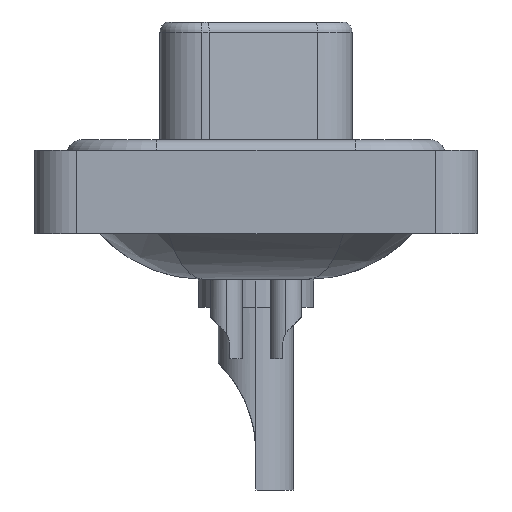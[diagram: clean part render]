
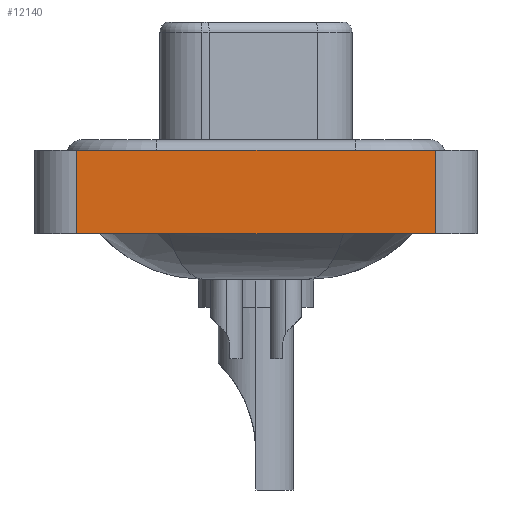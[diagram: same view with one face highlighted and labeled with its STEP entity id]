
A CAD part, left-side view. The second image highlights one B-rep face of the part: STEP entity #12140.
In plain terms, the highlighted planar face has unit normal (-1, 0, 0).
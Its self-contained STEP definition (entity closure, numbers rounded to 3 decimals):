
#59 = CARTESIAN_POINT ( 'NONE',  ( -7.25, 8.55, -3.6 ) ) ;
#99 = CARTESIAN_POINT ( 'NONE',  ( -7.25, 8.55, 0.4 ) ) ;
#453 = ORIENTED_EDGE ( 'NONE', *, *, #15666, .F. ) ;
#729 = CARTESIAN_POINT ( 'NONE',  ( -7.25, -8.55, -3.6 ) ) ;
#857 = CARTESIAN_POINT ( 'NONE',  ( -7.25, -8.55, -3.6 ) ) ;
#1236 = LINE ( 'NONE', #14995, #11742 ) ;
#2624 = DIRECTION ( 'NONE',  ( 0., 0., 1. ) ) ;
#2894 = CARTESIAN_POINT ( 'NONE',  ( -7.25, -8.55, -3.6 ) ) ;
#2936 = EDGE_CURVE ( 'NONE', #14469, #10672, #1236, .T. ) ;
#3471 = EDGE_CURVE ( 'NONE', #14469, #10369, #9196, .T. ) ;
#3780 = DIRECTION ( 'NONE',  ( 0., -1., 0. ) ) ;
#5906 = EDGE_LOOP ( 'NONE', ( #14948, #453, #14225, #9533 ) ) ;
#6385 = DIRECTION ( 'NONE',  ( 0., 0., 1. ) ) ;
#7827 = DIRECTION ( 'NONE',  ( 0., 0., 1. ) ) ;
#8019 = CARTESIAN_POINT ( 'NONE',  ( -7.25, 8.55, -3.6 ) ) ;
#8246 = VERTEX_POINT ( 'NONE', #10189 ) ;
#8481 = EDGE_CURVE ( 'NONE', #10672, #8246, #13263, .T. ) ;
#9196 = LINE ( 'NONE', #8019, #16309 ) ;
#9533 = ORIENTED_EDGE ( 'NONE', *, *, #2936, .T. ) ;
#10189 = CARTESIAN_POINT ( 'NONE',  ( -7.25, -8.55, 0.4 ) ) ;
#10369 = VERTEX_POINT ( 'NONE', #99 ) ;
#10672 = VERTEX_POINT ( 'NONE', #729 ) ;
#11132 = AXIS2_PLACEMENT_3D ( 'NONE', #2894, #17854, #2624 ) ;
#11742 = VECTOR ( 'NONE', #3780, 1000. ) ;
#12140 = ADVANCED_FACE ( 'NONE', ( #15209 ), #13854, .T. ) ;
#13192 = CARTESIAN_POINT ( 'NONE',  ( -7.25, -8.55, 0.4 ) ) ;
#13263 = LINE ( 'NONE', #857, #15079 ) ;
#13854 = PLANE ( 'NONE',  #11132 ) ;
#14179 = DIRECTION ( 'NONE',  ( 0., -1., 0. ) ) ;
#14225 = ORIENTED_EDGE ( 'NONE', *, *, #3471, .F. ) ;
#14447 = LINE ( 'NONE', #13192, #17102 ) ;
#14469 = VERTEX_POINT ( 'NONE', #59 ) ;
#14948 = ORIENTED_EDGE ( 'NONE', *, *, #8481, .T. ) ;
#14995 = CARTESIAN_POINT ( 'NONE',  ( -7.25, -8.55, -3.6 ) ) ;
#15079 = VECTOR ( 'NONE', #6385, 1000. ) ;
#15209 = FACE_OUTER_BOUND ( 'NONE', #5906, .T. ) ;
#15666 = EDGE_CURVE ( 'NONE', #10369, #8246, #14447, .T. ) ;
#16309 = VECTOR ( 'NONE', #7827, 1000. ) ;
#17102 = VECTOR ( 'NONE', #14179, 1000. ) ;
#17854 = DIRECTION ( 'NONE',  ( -1., 0., 0. ) ) ;
